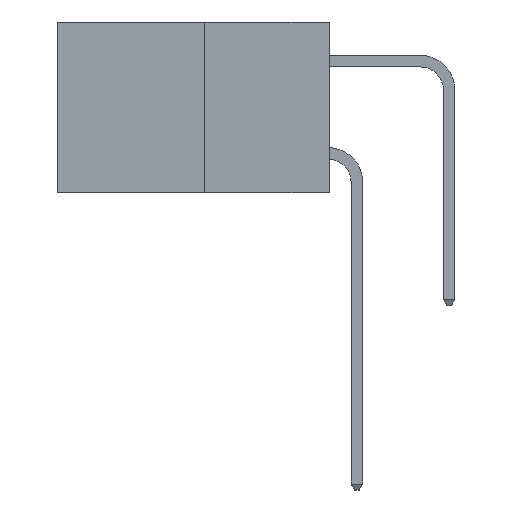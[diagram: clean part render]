
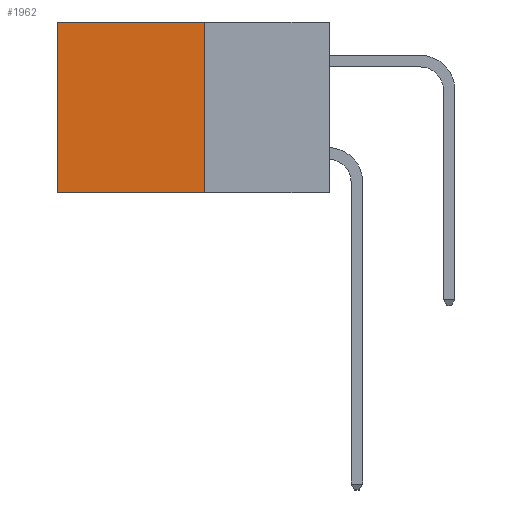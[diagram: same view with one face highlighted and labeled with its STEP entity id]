
A CAD part, left-side view. The second image highlights one B-rep face of the part: STEP entity #1962.
In plain terms, the highlighted planar face has unit normal (-1, 0, 0).
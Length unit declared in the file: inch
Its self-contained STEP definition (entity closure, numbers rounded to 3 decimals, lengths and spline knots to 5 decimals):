
#591 = CARTESIAN_POINT ( 'NONE',  ( 0.277, 0.27, 0. ) ) ;
#1556 = DIRECTION ( 'NONE',  ( 0., 1., 0. ) ) ;
#1939 = LINE ( 'NONE', #2203, #5860 ) ;
#1962 = ADVANCED_FACE ( 'NONE', ( #7973 ), #9914, .F. ) ;
#2009 = DIRECTION ( 'NONE',  ( 0., 0., -1. ) ) ;
#2203 = CARTESIAN_POINT ( 'NONE',  ( 0.277, 0.27, -0.37 ) ) ;
#2425 = LINE ( 'NONE', #3592, #10147 ) ;
#3511 = EDGE_CURVE ( 'NONE', #6200, #10820, #8746, .T. ) ;
#3592 = CARTESIAN_POINT ( 'NONE',  ( 0.277, 0.59, -0.37 ) ) ;
#4474 = VECTOR ( 'NONE', #1556, 39.37008 ) ;
#4618 = CARTESIAN_POINT ( 'NONE',  ( 0.277, 0.59, 0. ) ) ;
#4708 = AXIS2_PLACEMENT_3D ( 'NONE', #10877, #10613, #5676 ) ;
#4852 = EDGE_CURVE ( 'NONE', #9524, #6200, #1939, .T. ) ;
#5203 = CARTESIAN_POINT ( 'NONE',  ( 0.277, 0.59, -0.37 ) ) ;
#5676 = DIRECTION ( 'NONE',  ( 0., 0., -1. ) ) ;
#5828 = ORIENTED_EDGE ( 'NONE', *, *, #7979, .T. ) ;
#5860 = VECTOR ( 'NONE', #2009, 39.37008 ) ;
#6022 = ORIENTED_EDGE ( 'NONE', *, *, #3511, .F. ) ;
#6200 = VERTEX_POINT ( 'NONE', #8965 ) ;
#6419 = ORIENTED_EDGE ( 'NONE', *, *, #4852, .F. ) ;
#6470 = VECTOR ( 'NONE', #7433, 39.37008 ) ;
#6548 = ORIENTED_EDGE ( 'NONE', *, *, #9545, .T. ) ;
#6664 = VERTEX_POINT ( 'NONE', #4618 ) ;
#6852 = LINE ( 'NONE', #7748, #4474 ) ;
#7179 = EDGE_LOOP ( 'NONE', ( #5828, #6022, #6419, #6548 ) ) ;
#7433 = DIRECTION ( 'NONE',  ( 0., 1., 0. ) ) ;
#7450 = CARTESIAN_POINT ( 'NONE',  ( 0.277, 0.27, -0.37 ) ) ;
#7748 = CARTESIAN_POINT ( 'NONE',  ( 0.277, 0.27, 0. ) ) ;
#7973 = FACE_OUTER_BOUND ( 'NONE', #7179, .T. ) ;
#7979 = EDGE_CURVE ( 'NONE', #6664, #10820, #2425, .T. ) ;
#8746 = LINE ( 'NONE', #7450, #6470 ) ;
#8965 = CARTESIAN_POINT ( 'NONE',  ( 0.277, 0.27, -0.37 ) ) ;
#9524 = VERTEX_POINT ( 'NONE', #591 ) ;
#9545 = EDGE_CURVE ( 'NONE', #9524, #6664, #6852, .T. ) ;
#9635 = DIRECTION ( 'NONE',  ( 0., 0., -1. ) ) ;
#9914 = PLANE ( 'NONE',  #4708 ) ;
#10147 = VECTOR ( 'NONE', #9635, 39.37008 ) ;
#10613 = DIRECTION ( 'NONE',  ( 1., 0., 0. ) ) ;
#10820 = VERTEX_POINT ( 'NONE', #5203 ) ;
#10877 = CARTESIAN_POINT ( 'NONE',  ( 0.277, 0.27, -0.37 ) ) ;
